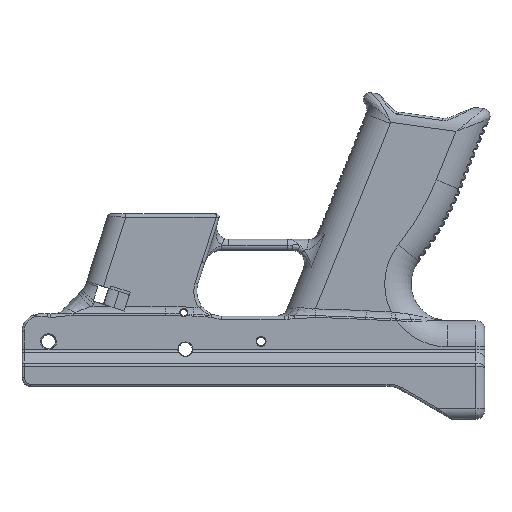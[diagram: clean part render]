
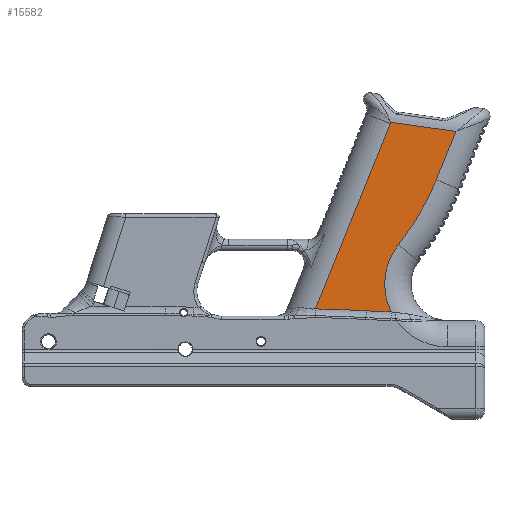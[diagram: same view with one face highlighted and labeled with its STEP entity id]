
A CAD part, front view. The second image highlights one B-rep face of the part: STEP entity #15582.
In plain terms, the highlighted planar face has unit normal (0, -1, 0).
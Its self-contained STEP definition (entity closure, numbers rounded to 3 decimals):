
#1522=PLANE('',#17182);
#2761=FACE_OUTER_BOUND('',#3764,.T.);
#3764=EDGE_LOOP('',(#14515,#14516,#14517,#14518,#14519,#14520,#14521,#14522));
#3896=LINE('',#21784,#4707);
#4145=LINE('',#32319,#4956);
#4589=LINE('',#41160,#5400);
#4707=VECTOR('',#17511,10.);
#4956=VECTOR('',#19080,10.);
#5400=VECTOR('',#21162,10.);
#5716=CIRCLE('',#16378,118.894);
#6118=CIRCLE('',#17157,689.416);
#6120=CIRCLE('',#17160,696.304);
#6135=CIRCLE('',#17183,28.63);
#6136=CIRCLE('',#17184,17.);
#6252=VERTEX_POINT('',#21781);
#6253=VERTEX_POINT('',#21783);
#6792=VERTEX_POINT('',#32311);
#6793=VERTEX_POINT('',#32318);
#6794=VERTEX_POINT('',#32335);
#7506=VERTEX_POINT('',#40711);
#7507=VERTEX_POINT('',#40718);
#7514=VERTEX_POINT('',#41159);
#7677=EDGE_CURVE('',#6252,#6253,#3896,.T.);
#8608=EDGE_CURVE('',#6792,#6793,#4145,.T.);
#8612=EDGE_CURVE('',#6253,#6794,#5716,.T.);
#9835=EDGE_CURVE('',#7506,#7507,#6118,.T.);
#9837=EDGE_CURVE('',#7507,#6792,#6120,.T.);
#9859=EDGE_CURVE('',#6794,#7506,#6135,.T.);
#9860=EDGE_CURVE('',#7514,#6252,#4589,.T.);
#9861=EDGE_CURVE('',#6793,#7514,#6136,.T.);
#14515=ORIENTED_EDGE('',*,*,#9835,.F.);
#14516=ORIENTED_EDGE('',*,*,#9859,.F.);
#14517=ORIENTED_EDGE('',*,*,#8612,.F.);
#14518=ORIENTED_EDGE('',*,*,#7677,.F.);
#14519=ORIENTED_EDGE('',*,*,#9860,.F.);
#14520=ORIENTED_EDGE('',*,*,#9861,.F.);
#14521=ORIENTED_EDGE('',*,*,#8608,.F.);
#14522=ORIENTED_EDGE('',*,*,#9837,.F.);
#15582=ADVANCED_FACE('',(#2761),#1522,.T.);
#16378=AXIS2_PLACEMENT_3D('',#32336,#19109,#19110);
#17157=AXIS2_PLACEMENT_3D('',#40719,#21108,#21109);
#17160=AXIS2_PLACEMENT_3D('',#40722,#21114,#21115);
#17182=AXIS2_PLACEMENT_3D('',#41157,#21158,#21159);
#17183=AXIS2_PLACEMENT_3D('',#41158,#21160,#21161);
#17184=AXIS2_PLACEMENT_3D('',#41161,#21163,#21164);
#17511=DIRECTION('',(-0.375,0.,-0.927));
#19080=DIRECTION('',(0.375,0.,0.927));
#19109=DIRECTION('center_axis',(0.,1.,0.));
#19110=DIRECTION('ref_axis',(0.891,0.,-0.454));
#21108=DIRECTION('center_axis',(0.,1.,0.));
#21109=DIRECTION('ref_axis',(0.037,0.,0.999));
#21114=DIRECTION('center_axis',(0.,-1.,0.));
#21115=DIRECTION('ref_axis',(-0.054,0.,-0.999));
#21158=DIRECTION('center_axis',(0.,-1.,0.));
#21159=DIRECTION('ref_axis',(1.,0.,0.));
#21160=DIRECTION('center_axis',(0.,-1.,0.));
#21161=DIRECTION('ref_axis',(0.782,0.,-0.624));
#21162=DIRECTION('',(0.99,0.,-0.139));
#21163=DIRECTION('center_axis',(0.,-1.,0.));
#21164=DIRECTION('ref_axis',(0.992,0.,0.126));
#21781=CARTESIAN_POINT('',(117.841,-14.625,19.236));
#21783=CARTESIAN_POINT('',(108.893,-14.625,-2.912));
#21784=CARTESIAN_POINT('',(111.761,-14.625,4.188));
#32311=CARTESIAN_POINT('',(53.832,-14.625,-61.703));
#32318=CARTESIAN_POINT('',(87.937,-14.625,22.71));
#32319=CARTESIAN_POINT('',(70.22,-14.625,-21.141));
#32335=CARTESIAN_POINT('',(91.6,-14.625,-32.517));
#32336=CARTESIAN_POINT('Origin',(-1.344,-14.625,41.627));
#40711=CARTESIAN_POINT('',(88.326,-14.625,-63.079));
#40718=CARTESIAN_POINT('',(76.954,-14.625,-62.561));
#40719=CARTESIAN_POINT('Origin',(113.981,-14.625,625.86));
#40722=CARTESIAN_POINT('Origin',(39.557,-14.625,-757.86));
#41157=CARTESIAN_POINT('Origin',(86.464,-14.625,-15.081));
#41158=CARTESIAN_POINT('Origin',(113.981,-14.625,-50.37));
#41159=CARTESIAN_POINT('',(88.199,-14.625,23.402));
#41160=CARTESIAN_POINT('',(84.577,-14.625,23.911));
#41161=CARTESIAN_POINT('Origin',(72.175,-14.625,29.078));
